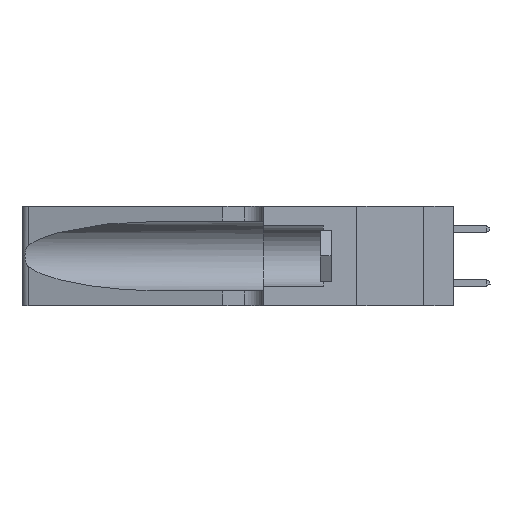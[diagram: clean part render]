
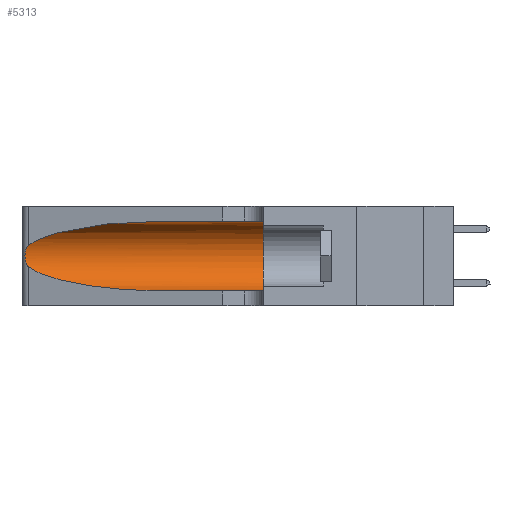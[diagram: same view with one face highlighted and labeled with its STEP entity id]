
A CAD part, left-side view. The second image highlights one B-rep face of the part: STEP entity #5313.
In plain terms, the highlighted cylindrical face has radius 3.308 mm (diameter 6.617 mm), a partial arc.
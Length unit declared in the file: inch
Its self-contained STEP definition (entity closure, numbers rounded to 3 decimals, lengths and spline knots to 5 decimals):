
#327 = DIRECTION ( 'NONE',  ( 0., -1., 0. ) ) ;
#678 = DIRECTION ( 'NONE',  ( 0., 1., 0. ) ) ;
#933 = AXIS2_PLACEMENT_3D ( 'NONE', #9909, #678, #11433 ) ;
#2193 = CARTESIAN_POINT ( 'NONE',  ( 0.25787, 1.23484, 0.2124 ) ) ;
#2330 =( BOUNDED_CURVE ( )  B_SPLINE_CURVE ( 3, ( #5402, #13003, #9971, #16023 ),
 .UNSPECIFIED., .F., .F. ) 
 B_SPLINE_CURVE_WITH_KNOTS ( ( 4, 4 ),
 ( 3.44316, 4.71239 ),
 .UNSPECIFIED. ) 
 CURVE ( )  GEOMETRIC_REPRESENTATION_ITEM ( )  RATIONAL_B_SPLINE_CURVE ( ( 1., 0.87, 0.87, 1. ) ) 
 REPRESENTATION_ITEM ( '' )  );
#2344 = EDGE_CURVE ( 'NONE', #12260, #16229, #4351, .T. ) ;
#2528 = ORIENTED_EDGE ( 'NONE', *, *, #17620, .F. ) ;
#2569 = ORIENTED_EDGE ( 'NONE', *, *, #3373, .T. ) ;
#2753 = DIRECTION ( 'NONE',  ( 0., -1., 0. ) ) ;
#3373 = EDGE_CURVE ( 'NONE', #10473, #7116, #2330, .T. ) ;
#3777 = CARTESIAN_POINT ( 'NONE',  ( 0.26018, 1.23835, 0.19895 ) ) ;
#4004 = CARTESIAN_POINT ( 'NONE',  ( 0.1305, 1.61858, 0.185 ) ) ;
#4078 = EDGE_CURVE ( 'NONE', #12260, #14199, #15685, .T. ) ;
#4351 =( BOUNDED_CURVE ( )  B_SPLINE_CURVE ( 3, ( #15689, #13465, #13289, #9400 ),
 .UNSPECIFIED., .F., .F. ) 
 B_SPLINE_CURVE_WITH_KNOTS ( ( 4, 4 ),
 ( 1.5708, 2.84003 ),
 .UNSPECIFIED. ) 
 CURVE ( )  GEOMETRIC_REPRESENTATION_ITEM ( )  RATIONAL_B_SPLINE_CURVE ( ( 1., 0.87, 0.87, 1. ) ) 
 REPRESENTATION_ITEM ( '' )  );
#5146 = ORIENTED_EDGE ( 'NONE', *, *, #2344, .T. ) ;
#5312 = CARTESIAN_POINT ( 'NONE',  ( 0.26075, 1.23896, 0.178 ) ) ;
#5313 = ADVANCED_FACE ( 'NONE', ( #9512 ), #13054, .F. ) ;
#5395 = ORIENTED_EDGE ( 'NONE', *, *, #16260, .T. ) ;
#5402 = CARTESIAN_POINT ( 'NONE',  ( 0.25487, 1.22718, 0.14631 ) ) ;
#5709 = VECTOR ( 'NONE', #327, 39.37008 ) ;
#6860 = CARTESIAN_POINT ( 'NONE',  ( 0.25856, 1.23593, 0.16098 ) ) ;
#7093 = DIRECTION ( 'NONE',  ( 0., -1., 0. ) ) ;
#7116 = VERTEX_POINT ( 'NONE', #8805 ) ;
#7166 = VECTOR ( 'NONE', #2753, 39.37008 ) ;
#8377 = CARTESIAN_POINT ( 'NONE',  ( 0.25555, 1.22994, 0.2215 ) ) ;
#8442 = CARTESIAN_POINT ( 'NONE',  ( 0.25639, 1.23186, 0.15144 ) ) ;
#8805 = CARTESIAN_POINT ( 'NONE',  ( 0.1305, 0.72297, 0.05475 ) ) ;
#9400 = CARTESIAN_POINT ( 'NONE',  ( 0.25487, 1.22718, 0.22369 ) ) ;
#9512 = FACE_OUTER_BOUND ( 'NONE', #14797, .T. ) ;
#9714 = EDGE_CURVE ( 'NONE', #7116, #18046, #17276, .T. ) ;
#9909 = CARTESIAN_POINT ( 'NONE',  ( 0.1305, 0.35, 0.185 ) ) ;
#9950 = CARTESIAN_POINT ( 'NONE',  ( 0.25487, 1.22718, 0.14631 ) ) ;
#9971 = CARTESIAN_POINT ( 'NONE',  ( 0.18966, 0.96281, 0.05475 ) ) ;
#10258 = CIRCLE ( 'NONE', #933, 0.13025 ) ;
#10473 = VERTEX_POINT ( 'NONE', #11595 ) ;
#11090 = CARTESIAN_POINT ( 'NONE',  ( 0.1305, 1.61858, 0.05475 ) ) ;
#11414 = CARTESIAN_POINT ( 'NONE',  ( 0.25639, 1.23184, 0.21858 ) ) ;
#11433 = DIRECTION ( 'NONE',  ( 0., 0., 1. ) ) ;
#11595 = CARTESIAN_POINT ( 'NONE',  ( 0.25487, 1.22718, 0.14631 ) ) ;
#12260 = VERTEX_POINT ( 'NONE', #16211 ) ;
#12915 = CARTESIAN_POINT ( 'NONE',  ( 0.25854, 1.2359, 0.20912 ) ) ;
#13003 = CARTESIAN_POINT ( 'NONE',  ( 0.2373, 1.15595, 0.08982 ) ) ;
#13054 = CYLINDRICAL_SURFACE ( 'NONE', #18660, 0.13025 ) ;
#13157 = CARTESIAN_POINT ( 'NONE',  ( 0.1305, 0.35, 0.05475 ) ) ;
#13289 = CARTESIAN_POINT ( 'NONE',  ( 0.2373, 1.15595, 0.28018 ) ) ;
#13465 = CARTESIAN_POINT ( 'NONE',  ( 0.18966, 0.96281, 0.31525 ) ) ;
#13593 = ORIENTED_EDGE ( 'NONE', *, *, #9714, .T. ) ;
#14199 = VERTEX_POINT ( 'NONE', #19510 ) ;
#14433 = CARTESIAN_POINT ( 'NONE',  ( 0.26075, 1.23896, 0.19203 ) ) ;
#14797 = EDGE_LOOP ( 'NONE', ( #5146, #5395, #2569, #13593, #2528, #18762 ) ) ;
#15685 = LINE ( 'NONE', #17871, #7166 ) ;
#15689 = CARTESIAN_POINT ( 'NONE',  ( 0.1305, 0.72297, 0.31525 ) ) ;
#15944 = CARTESIAN_POINT ( 'NONE',  ( 0.26017, 1.23833, 0.17102 ) ) ;
#16023 = CARTESIAN_POINT ( 'NONE',  ( 0.1305, 0.72297, 0.05475 ) ) ;
#16211 = CARTESIAN_POINT ( 'NONE',  ( 0.1305, 0.72297, 0.31525 ) ) ;
#16229 = VERTEX_POINT ( 'NONE', #17281 ) ;
#16260 = EDGE_CURVE ( 'NONE', #16229, #10473, #18506, .T. ) ;
#17276 = LINE ( 'NONE', #11090, #5709 ) ;
#17281 = CARTESIAN_POINT ( 'NONE',  ( 0.25487, 1.22718, 0.22369 ) ) ;
#17411 = CARTESIAN_POINT ( 'NONE',  ( 0.25789, 1.23486, 0.15765 ) ) ;
#17620 = EDGE_CURVE ( 'NONE', #14199, #18046, #10258, .T. ) ;
#17632 = DIRECTION ( 'NONE',  ( 0., 0., -1. ) ) ;
#17871 = CARTESIAN_POINT ( 'NONE',  ( 0.1305, 1.61858, 0.31525 ) ) ;
#18046 = VERTEX_POINT ( 'NONE', #13157 ) ;
#18506 = B_SPLINE_CURVE_WITH_KNOTS ( 'NONE', 3,
 ( #18845, #8377, #11414, #2193, #12915, #3777, #14433, #5312, #15944, #6860, #17411, #8442, #18913, #9950 ),
 .UNSPECIFIED., .F., .F.,
 ( 4, 2, 2, 2, 2, 2, 4 ),
 ( 0., 0.00027, 0.00053, 0.00107, 0.0016, 0.00187, 0.00214 ),
 .UNSPECIFIED. ) ;
#18660 = AXIS2_PLACEMENT_3D ( 'NONE', #4004, #7093, #17632 ) ;
#18762 = ORIENTED_EDGE ( 'NONE', *, *, #4078, .F. ) ;
#18845 = CARTESIAN_POINT ( 'NONE',  ( 0.25487, 1.22718, 0.22369 ) ) ;
#18913 = CARTESIAN_POINT ( 'NONE',  ( 0.25555, 1.22993, 0.14849 ) ) ;
#19510 = CARTESIAN_POINT ( 'NONE',  ( 0.1305, 0.35, 0.31525 ) ) ;
